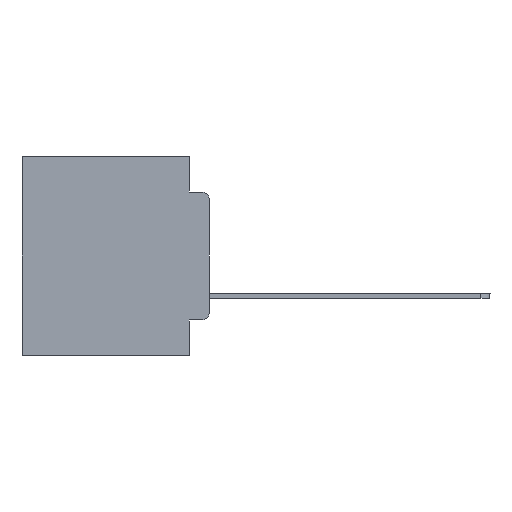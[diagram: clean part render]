
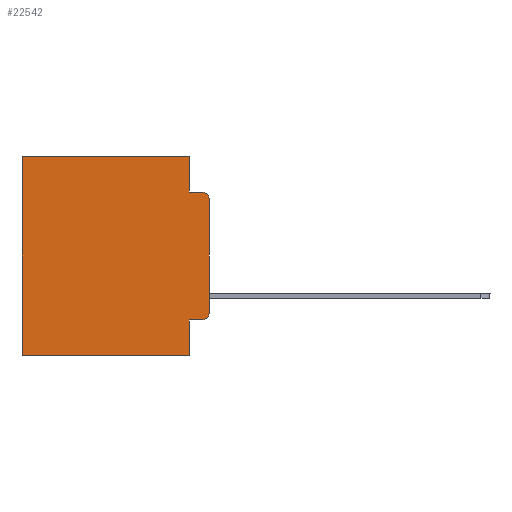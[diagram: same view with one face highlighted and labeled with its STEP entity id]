
A CAD part, left-side view. The second image highlights one B-rep face of the part: STEP entity #22542.
In plain terms, the highlighted planar face has unit normal (-1, 0, 0).
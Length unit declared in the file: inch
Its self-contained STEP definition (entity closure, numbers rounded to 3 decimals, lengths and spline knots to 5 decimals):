
#442 = CARTESIAN_POINT ( 'NONE',  ( 0.298, 0.051, 0. ) ) ;
#673 = LINE ( 'NONE', #442, #6850 ) ;
#802 = VECTOR ( 'NONE', #2154, 39.37008 ) ;
#872 = EDGE_CURVE ( 'NONE', #19777, #19487, #6630, .T. ) ;
#1936 = CARTESIAN_POINT ( 'NONE',  ( 0.298, 0.02, -0.4115 ) ) ;
#2154 = DIRECTION ( 'NONE',  ( 0., 0., -1. ) ) ;
#2320 = CARTESIAN_POINT ( 'NONE',  ( 0.298, 0., 0. ) ) ;
#2534 = ORIENTED_EDGE ( 'NONE', *, *, #7234, .T. ) ;
#2919 = VECTOR ( 'NONE', #5374, 39.37008 ) ;
#3511 = CARTESIAN_POINT ( 'NONE',  ( 0.298, 0.051, -0.4115 ) ) ;
#3780 = DIRECTION ( 'NONE',  ( 0., -1., 0. ) ) ;
#4648 = EDGE_CURVE ( 'NONE', #7560, #19777, #13249, .T. ) ;
#5070 = CARTESIAN_POINT ( 'NONE',  ( 0.298, 0.02, -0.0885 ) ) ;
#5095 = ORIENTED_EDGE ( 'NONE', *, *, #21488, .F. ) ;
#5261 = DIRECTION ( 'NONE',  ( 0., -1., 0. ) ) ;
#5374 = DIRECTION ( 'NONE',  ( 0., 1., 0. ) ) ;
#5941 = CARTESIAN_POINT ( 'NONE',  ( 0.298, 0.02, -0.1085 ) ) ;
#5960 = VECTOR ( 'NONE', #3780, 39.37008 ) ;
#6130 = CARTESIAN_POINT ( 'NONE',  ( 0.298, 0.051, -0.5 ) ) ;
#6204 = AXIS2_PLACEMENT_3D ( 'NONE', #6996, #26627, #6729 ) ;
#6630 = LINE ( 'NONE', #10692, #802 ) ;
#6723 = DIRECTION ( 'NONE',  ( 0., 0., -1. ) ) ;
#6729 = DIRECTION ( 'NONE',  ( 0., 0., -1. ) ) ;
#6850 = VECTOR ( 'NONE', #20147, 39.37008 ) ;
#6996 = CARTESIAN_POINT ( 'NONE',  ( 0.298, 0., 0. ) ) ;
#7074 = VECTOR ( 'NONE', #5261, 39.37008 ) ;
#7234 = EDGE_CURVE ( 'NONE', #18691, #11113, #7943, .T. ) ;
#7398 = VECTOR ( 'NONE', #11520, 39.37008 ) ;
#7560 = VERTEX_POINT ( 'NONE', #11703 ) ;
#7943 = CIRCLE ( 'NONE', #17775, 0.02 ) ;
#8426 = ORIENTED_EDGE ( 'NONE', *, *, #15763, .F. ) ;
#8952 = CARTESIAN_POINT ( 'NONE',  ( 0.298, 0., -0.3915 ) ) ;
#9388 = LINE ( 'NONE', #3511, #5960 ) ;
#9510 = EDGE_CURVE ( 'NONE', #27337, #15784, #23243, .T. ) ;
#9825 = CARTESIAN_POINT ( 'NONE',  ( 0.298, 0.051, -0.0885 ) ) ;
#10692 = CARTESIAN_POINT ( 'NONE',  ( 0.298, 0.473, 0. ) ) ;
#11113 = VERTEX_POINT ( 'NONE', #8952 ) ;
#11520 = DIRECTION ( 'NONE',  ( 0., 1., 0. ) ) ;
#11703 = CARTESIAN_POINT ( 'NONE',  ( 0.298, 0.051, 0. ) ) ;
#12087 = LINE ( 'NONE', #14169, #26478 ) ;
#12255 = DIRECTION ( 'NONE',  ( -1., 0., 0. ) ) ;
#12445 = VECTOR ( 'NONE', #6723, 39.37008 ) ;
#12841 = EDGE_CURVE ( 'NONE', #7560, #20859, #12087, .T. ) ;
#13249 = LINE ( 'NONE', #26910, #7398 ) ;
#13438 = PLANE ( 'NONE',  #6204 ) ;
#13613 = CARTESIAN_POINT ( 'NONE',  ( 0.298, 0.473, -0.5 ) ) ;
#13890 = LINE ( 'NONE', #27258, #2919 ) ;
#14169 = CARTESIAN_POINT ( 'NONE',  ( 0.298, 0.051, 0. ) ) ;
#14309 = CARTESIAN_POINT ( 'NONE',  ( 0.298, 0.051, -0.4115 ) ) ;
#14973 = CARTESIAN_POINT ( 'NONE',  ( 0.298, 0.473, 0. ) ) ;
#15763 = EDGE_CURVE ( 'NONE', #20859, #15784, #19406, .T. ) ;
#15784 = VERTEX_POINT ( 'NONE', #5070 ) ;
#16685 = DIRECTION ( 'NONE',  ( 0., 0., -1. ) ) ;
#16760 = DIRECTION ( 'NONE',  ( -1., 0., 0. ) ) ;
#17775 = AXIS2_PLACEMENT_3D ( 'NONE', #18831, #16760, #19208 ) ;
#18691 = VERTEX_POINT ( 'NONE', #1936 ) ;
#18772 = ORIENTED_EDGE ( 'NONE', *, *, #4648, .T. ) ;
#18831 = CARTESIAN_POINT ( 'NONE',  ( 0.298, 0.02, -0.3915 ) ) ;
#19208 = DIRECTION ( 'NONE',  ( 0., 0., -1. ) ) ;
#19406 = LINE ( 'NONE', #20650, #7074 ) ;
#19487 = VERTEX_POINT ( 'NONE', #13613 ) ;
#19777 = VERTEX_POINT ( 'NONE', #14973 ) ;
#20147 = DIRECTION ( 'NONE',  ( 0., 0., -1. ) ) ;
#20650 = CARTESIAN_POINT ( 'NONE',  ( 0.298, 0.051, -0.0885 ) ) ;
#20859 = VERTEX_POINT ( 'NONE', #9825 ) ;
#21488 = EDGE_CURVE ( 'NONE', #26920, #19487, #13890, .T. ) ;
#21568 = ORIENTED_EDGE ( 'NONE', *, *, #24477, .F. ) ;
#22074 = ORIENTED_EDGE ( 'NONE', *, *, #26080, .F. ) ;
#22162 = EDGE_LOOP ( 'NONE', ( #21568, #25358, #8426, #24131, #18772, #23935, #5095, #22074, #27729, #2534 ) ) ;
#22356 = LINE ( 'NONE', #2320, #12445 ) ;
#22542 = ADVANCED_FACE ( 'NONE', ( #23137 ), #13438, .F. ) ;
#23137 = FACE_OUTER_BOUND ( 'NONE', #22162, .T. ) ;
#23149 = DIRECTION ( 'NONE',  ( 0., 0., -1. ) ) ;
#23243 = CIRCLE ( 'NONE', #26087, 0.02 ) ;
#23935 = ORIENTED_EDGE ( 'NONE', *, *, #872, .T. ) ;
#24131 = ORIENTED_EDGE ( 'NONE', *, *, #12841, .F. ) ;
#24172 = EDGE_CURVE ( 'NONE', #25050, #18691, #9388, .T. ) ;
#24477 = EDGE_CURVE ( 'NONE', #27337, #11113, #22356, .T. ) ;
#25050 = VERTEX_POINT ( 'NONE', #14309 ) ;
#25358 = ORIENTED_EDGE ( 'NONE', *, *, #9510, .T. ) ;
#26080 = EDGE_CURVE ( 'NONE', #25050, #26920, #673, .T. ) ;
#26087 = AXIS2_PLACEMENT_3D ( 'NONE', #5941, #12255, #16685 ) ;
#26478 = VECTOR ( 'NONE', #23149, 39.37008 ) ;
#26627 = DIRECTION ( 'NONE',  ( 1., 0., 0. ) ) ;
#26910 = CARTESIAN_POINT ( 'NONE',  ( 0.298, 0., 0. ) ) ;
#26920 = VERTEX_POINT ( 'NONE', #6130 ) ;
#27258 = CARTESIAN_POINT ( 'NONE',  ( 0.298, 0., -0.5 ) ) ;
#27337 = VERTEX_POINT ( 'NONE', #27338 ) ;
#27338 = CARTESIAN_POINT ( 'NONE',  ( 0.298, 0., -0.1085 ) ) ;
#27729 = ORIENTED_EDGE ( 'NONE', *, *, #24172, .T. ) ;
